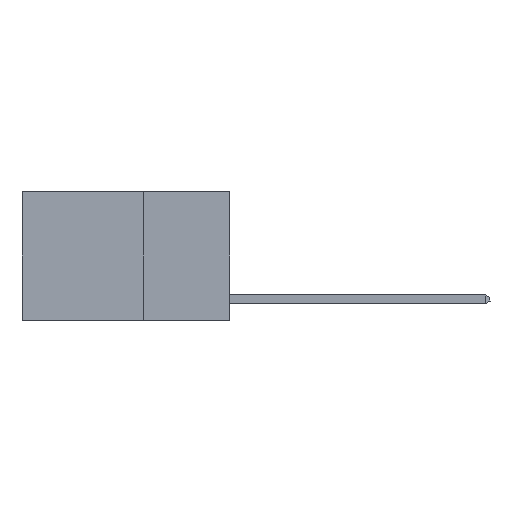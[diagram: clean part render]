
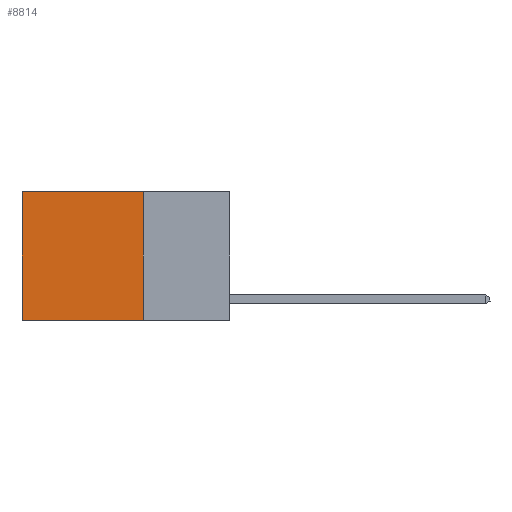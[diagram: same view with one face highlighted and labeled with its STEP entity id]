
A CAD part, left-side view. The second image highlights one B-rep face of the part: STEP entity #8814.
In plain terms, the highlighted planar face has unit normal (-1, 0, 0).
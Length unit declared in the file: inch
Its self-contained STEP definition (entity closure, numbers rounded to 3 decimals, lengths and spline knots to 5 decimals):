
#38 = CARTESIAN_POINT ( 'NONE',  ( 0.2625, 0.25, -0.37 ) ) ;
#253 = LINE ( 'NONE', #3834, #2818 ) ;
#302 = DIRECTION ( 'NONE',  ( 0., 0., -1. ) ) ;
#594 = DIRECTION ( 'NONE',  ( 1., 0., 0. ) ) ;
#670 = LINE ( 'NONE', #4103, #2700 ) ;
#988 = EDGE_CURVE ( 'NONE', #2377, #7666, #10216, .T. ) ;
#1594 = DIRECTION ( 'NONE',  ( 0., 1., 0. ) ) ;
#1682 = AXIS2_PLACEMENT_3D ( 'NONE', #14195, #594, #1862 ) ;
#1842 = ORIENTED_EDGE ( 'NONE', *, *, #2597, .F. ) ;
#1862 = DIRECTION ( 'NONE',  ( 0., 0., -1. ) ) ;
#2377 = VERTEX_POINT ( 'NONE', #15116 ) ;
#2393 = CARTESIAN_POINT ( 'NONE',  ( 0.2625, 0.6, -0.37 ) ) ;
#2597 = EDGE_CURVE ( 'NONE', #9780, #7666, #3468, .T. ) ;
#2700 = VECTOR ( 'NONE', #12770, 39.37008 ) ;
#2780 = ORIENTED_EDGE ( 'NONE', *, *, #988, .T. ) ;
#2818 = VECTOR ( 'NONE', #1594, 39.37008 ) ;
#2904 = FACE_OUTER_BOUND ( 'NONE', #10088, .T. ) ;
#3468 = LINE ( 'NONE', #38, #12437 ) ;
#3640 = EDGE_CURVE ( 'NONE', #5690, #9780, #670, .T. ) ;
#3834 = CARTESIAN_POINT ( 'NONE',  ( 0.2625, 0.25, 0. ) ) ;
#4103 = CARTESIAN_POINT ( 'NONE',  ( 0.2625, 0.25, 0. ) ) ;
#5530 = PLANE ( 'NONE',  #1682 ) ;
#5690 = VERTEX_POINT ( 'NONE', #15211 ) ;
#5942 = DIRECTION ( 'NONE',  ( 0., 1., 0. ) ) ;
#6367 = CARTESIAN_POINT ( 'NONE',  ( 0.2625, 0.6, 0. ) ) ;
#6937 = CARTESIAN_POINT ( 'NONE',  ( 0.2625, 0.25, -0.37 ) ) ;
#7666 = VERTEX_POINT ( 'NONE', #2393 ) ;
#8814 = ADVANCED_FACE ( 'NONE', ( #2904 ), #5530, .F. ) ;
#9780 = VERTEX_POINT ( 'NONE', #6937 ) ;
#10088 = EDGE_LOOP ( 'NONE', ( #2780, #1842, #11853, #14794 ) ) ;
#10216 = LINE ( 'NONE', #6367, #10512 ) ;
#10512 = VECTOR ( 'NONE', #302, 39.37008 ) ;
#11853 = ORIENTED_EDGE ( 'NONE', *, *, #3640, .F. ) ;
#12437 = VECTOR ( 'NONE', #5942, 39.37008 ) ;
#12770 = DIRECTION ( 'NONE',  ( 0., 0., -1. ) ) ;
#14195 = CARTESIAN_POINT ( 'NONE',  ( 0.2625, 0.25, 0. ) ) ;
#14794 = ORIENTED_EDGE ( 'NONE', *, *, #15126, .T. ) ;
#15116 = CARTESIAN_POINT ( 'NONE',  ( 0.2625, 0.6, 0. ) ) ;
#15126 = EDGE_CURVE ( 'NONE', #5690, #2377, #253, .T. ) ;
#15211 = CARTESIAN_POINT ( 'NONE',  ( 0.2625, 0.25, 0. ) ) ;
